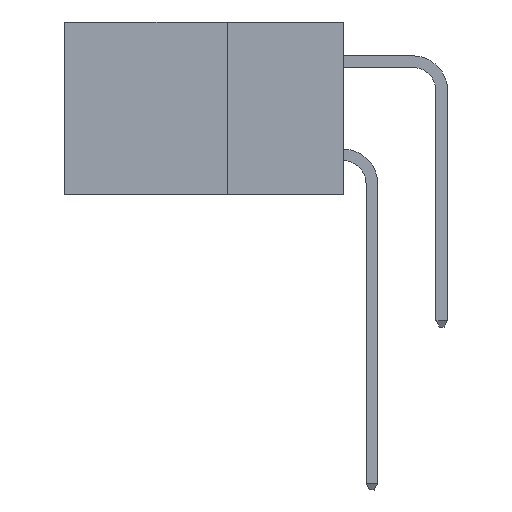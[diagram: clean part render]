
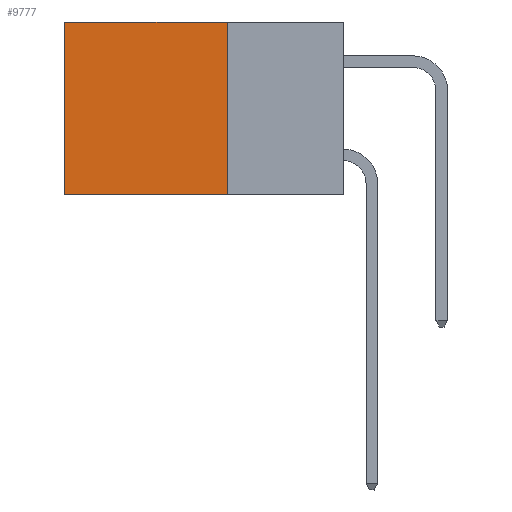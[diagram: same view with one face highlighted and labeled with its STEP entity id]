
A CAD part, left-side view. The second image highlights one B-rep face of the part: STEP entity #9777.
In plain terms, the highlighted planar face has unit normal (-1, 0, 0).
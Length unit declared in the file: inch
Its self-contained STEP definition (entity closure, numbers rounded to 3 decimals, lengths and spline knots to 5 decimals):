
#495 = LINE ( 'NONE', #22936, #15537 ) ;
#511 = VERTEX_POINT ( 'NONE', #25413 ) ;
#984 = VECTOR ( 'NONE', #23541, 39.37008 ) ;
#2650 = EDGE_LOOP ( 'NONE', ( #4831, #16094, #22759, #32271 ) ) ;
#2886 = CARTESIAN_POINT ( 'NONE',  ( 0.298, 0.25, 0. ) ) ;
#4831 = ORIENTED_EDGE ( 'NONE', *, *, #14743, .T. ) ;
#5484 = DIRECTION ( 'NONE',  ( 0., 0., -1. ) ) ;
#7872 = CARTESIAN_POINT ( 'NONE',  ( 0.298, 0.6, -0.37 ) ) ;
#9234 = EDGE_CURVE ( 'NONE', #11863, #9329, #495, .T. ) ;
#9329 = VERTEX_POINT ( 'NONE', #12807 ) ;
#9777 = ADVANCED_FACE ( 'NONE', ( #27699 ), #26642, .F. ) ;
#11195 = LINE ( 'NONE', #19196, #24669 ) ;
#11711 = CARTESIAN_POINT ( 'NONE',  ( 0.298, 0.25, 0. ) ) ;
#11863 = VERTEX_POINT ( 'NONE', #11711 ) ;
#12807 = CARTESIAN_POINT ( 'NONE',  ( 0.298, 0.25, -0.37 ) ) ;
#13938 = DIRECTION ( 'NONE',  ( 0., 1., 0. ) ) ;
#14444 = CARTESIAN_POINT ( 'NONE',  ( 0.298, 0.25, 0. ) ) ;
#14743 = EDGE_CURVE ( 'NONE', #511, #16756, #32679, .T. ) ;
#14787 = DIRECTION ( 'NONE',  ( 0., 1., 0. ) ) ;
#15537 = VECTOR ( 'NONE', #17393, 39.37008 ) ;
#16094 = ORIENTED_EDGE ( 'NONE', *, *, #16360, .F. ) ;
#16360 = EDGE_CURVE ( 'NONE', #9329, #16756, #11195, .T. ) ;
#16756 = VERTEX_POINT ( 'NONE', #7872 ) ;
#17393 = DIRECTION ( 'NONE',  ( 0., 0., -1. ) ) ;
#18582 = CARTESIAN_POINT ( 'NONE',  ( 0.298, 0.6, 0. ) ) ;
#19196 = CARTESIAN_POINT ( 'NONE',  ( 0.298, 0.25, -0.37 ) ) ;
#20386 = AXIS2_PLACEMENT_3D ( 'NONE', #2886, #21067, #5484 ) ;
#21067 = DIRECTION ( 'NONE',  ( 1., 0., 0. ) ) ;
#22759 = ORIENTED_EDGE ( 'NONE', *, *, #9234, .F. ) ;
#22936 = CARTESIAN_POINT ( 'NONE',  ( 0.298, 0.25, 0. ) ) ;
#23541 = DIRECTION ( 'NONE',  ( 0., 0., -1. ) ) ;
#24277 = EDGE_CURVE ( 'NONE', #11863, #511, #32921, .T. ) ;
#24428 = VECTOR ( 'NONE', #14787, 39.37008 ) ;
#24669 = VECTOR ( 'NONE', #13938, 39.37008 ) ;
#25413 = CARTESIAN_POINT ( 'NONE',  ( 0.298, 0.6, 0. ) ) ;
#26642 = PLANE ( 'NONE',  #20386 ) ;
#27699 = FACE_OUTER_BOUND ( 'NONE', #2650, .T. ) ;
#32271 = ORIENTED_EDGE ( 'NONE', *, *, #24277, .T. ) ;
#32679 = LINE ( 'NONE', #18582, #984 ) ;
#32921 = LINE ( 'NONE', #14444, #24428 ) ;
